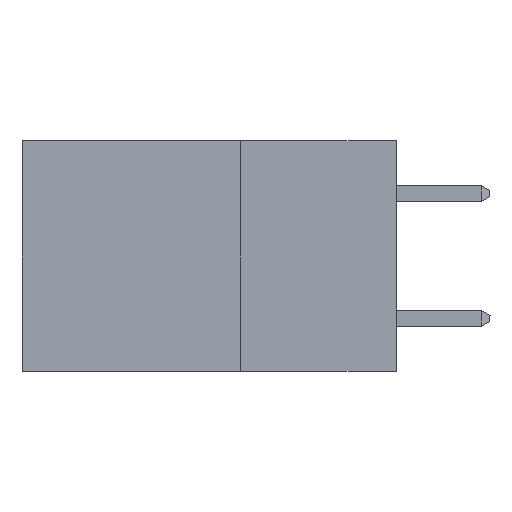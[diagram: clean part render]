
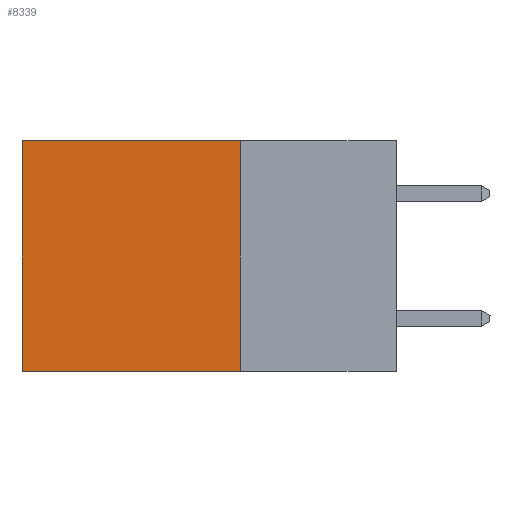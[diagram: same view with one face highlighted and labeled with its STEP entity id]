
A CAD part, left-side view. The second image highlights one B-rep face of the part: STEP entity #8339.
In plain terms, the highlighted planar face has unit normal (-1, 0, 0).
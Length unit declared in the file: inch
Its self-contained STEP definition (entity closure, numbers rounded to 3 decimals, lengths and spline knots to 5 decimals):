
#46 = VECTOR ( 'NONE', #1440, 39.37008 ) ;
#208 = VERTEX_POINT ( 'NONE', #829 ) ;
#829 = CARTESIAN_POINT ( 'NONE',  ( 0.2615, 0.6, 0. ) ) ;
#1408 = FACE_OUTER_BOUND ( 'NONE', #16406, .T. ) ;
#1440 = DIRECTION ( 'NONE',  ( 0., 1., 0. ) ) ;
#1479 = CARTESIAN_POINT ( 'NONE',  ( 0.2615, 0.25, -0.37 ) ) ;
#1666 = VECTOR ( 'NONE', #12592, 39.37008 ) ;
#2085 = VECTOR ( 'NONE', #4328, 39.37008 ) ;
#2309 = VERTEX_POINT ( 'NONE', #13210 ) ;
#2657 = VERTEX_POINT ( 'NONE', #16952 ) ;
#3286 = ORIENTED_EDGE ( 'NONE', *, *, #6675, .F. ) ;
#3315 = CARTESIAN_POINT ( 'NONE',  ( 0.2615, 0.25, -0.37 ) ) ;
#3901 = LINE ( 'NONE', #1479, #46 ) ;
#4328 = DIRECTION ( 'NONE',  ( 0., 1., 0. ) ) ;
#4500 = CARTESIAN_POINT ( 'NONE',  ( 0.2615, 0.25, -0.37 ) ) ;
#5344 = LINE ( 'NONE', #11213, #1666 ) ;
#5844 = PLANE ( 'NONE',  #12805 ) ;
#6675 = EDGE_CURVE ( 'NONE', #2657, #2309, #3901, .T. ) ;
#7175 = DIRECTION ( 'NONE',  ( 0., 0., -1. ) ) ;
#7734 = EDGE_CURVE ( 'NONE', #208, #2309, #5344, .T. ) ;
#7785 = EDGE_CURVE ( 'NONE', #17113, #2657, #14279, .T. ) ;
#8248 = CARTESIAN_POINT ( 'NONE',  ( 0.2615, 0.25, 0. ) ) ;
#8339 = ADVANCED_FACE ( 'NONE', ( #1408 ), #5844, .F. ) ;
#10261 = LINE ( 'NONE', #8248, #2085 ) ;
#11213 = CARTESIAN_POINT ( 'NONE',  ( 0.2615, 0.6, -0.37 ) ) ;
#12088 = ORIENTED_EDGE ( 'NONE', *, *, #7734, .T. ) ;
#12592 = DIRECTION ( 'NONE',  ( 0., 0., -1. ) ) ;
#12805 = AXIS2_PLACEMENT_3D ( 'NONE', #4500, #15099, #7175 ) ;
#13210 = CARTESIAN_POINT ( 'NONE',  ( 0.2615, 0.6, -0.37 ) ) ;
#14001 = DIRECTION ( 'NONE',  ( 0., 0., -1. ) ) ;
#14279 = LINE ( 'NONE', #3315, #17154 ) ;
#14337 = EDGE_CURVE ( 'NONE', #17113, #208, #10261, .T. ) ;
#14836 = ORIENTED_EDGE ( 'NONE', *, *, #14337, .T. ) ;
#15099 = DIRECTION ( 'NONE',  ( 1., 0., 0. ) ) ;
#15304 = ORIENTED_EDGE ( 'NONE', *, *, #7785, .F. ) ;
#16406 = EDGE_LOOP ( 'NONE', ( #12088, #3286, #15304, #14836 ) ) ;
#16695 = CARTESIAN_POINT ( 'NONE',  ( 0.2615, 0.25, 0. ) ) ;
#16952 = CARTESIAN_POINT ( 'NONE',  ( 0.2615, 0.25, -0.37 ) ) ;
#17113 = VERTEX_POINT ( 'NONE', #16695 ) ;
#17154 = VECTOR ( 'NONE', #14001, 39.37008 ) ;
